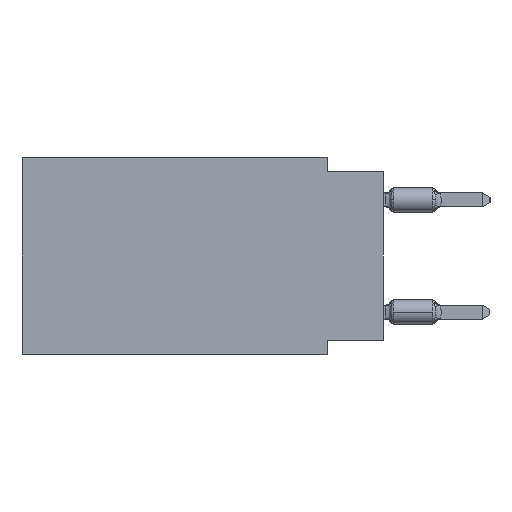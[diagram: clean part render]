
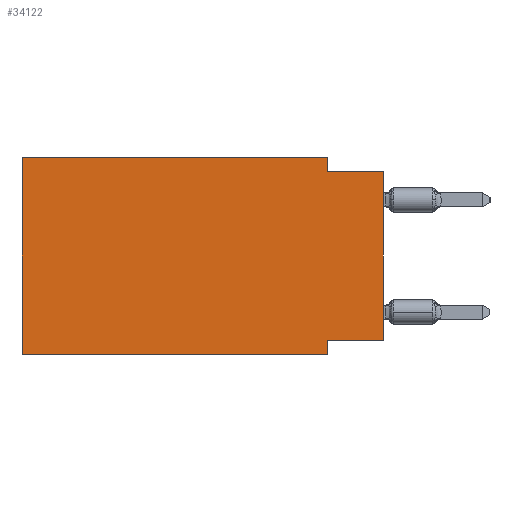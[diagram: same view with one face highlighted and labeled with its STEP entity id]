
A CAD part, left-side view. The second image highlights one B-rep face of the part: STEP entity #34122.
In plain terms, the highlighted planar face has unit normal (-1, 0, 0).
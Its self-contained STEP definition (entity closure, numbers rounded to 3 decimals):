
#1573 = DIRECTION ( 'NONE',  ( 0., 1., 0. ) ) ;
#1700 = ORIENTED_EDGE ( 'NONE', *, *, #41663, .F. ) ;
#1759 = CARTESIAN_POINT ( 'NONE',  ( 0., 0., -8.255 ) ) ;
#2011 = ORIENTED_EDGE ( 'NONE', *, *, #25797, .F. ) ;
#2292 = EDGE_CURVE ( 'NONE', #13753, #52711, #33575, .T. ) ;
#4711 = CARTESIAN_POINT ( 'NONE',  ( 0., 2.54, -8.255 ) ) ;
#5751 = EDGE_CURVE ( 'NONE', #40025, #49163, #55352, .T. ) ;
#7011 = CARTESIAN_POINT ( 'NONE',  ( 0., 2.54, -8.89 ) ) ;
#7287 = VECTOR ( 'NONE', #16326, 1000. ) ;
#8347 = VERTEX_POINT ( 'NONE', #1759 ) ;
#9127 = DIRECTION ( 'NONE',  ( 0., 0., 1. ) ) ;
#9453 = VECTOR ( 'NONE', #16396, 1000. ) ;
#9945 = CARTESIAN_POINT ( 'NONE',  ( 0., 0., -8.255 ) ) ;
#10442 = EDGE_CURVE ( 'NONE', #44852, #52711, #16675, .T. ) ;
#10452 = CARTESIAN_POINT ( 'NONE',  ( 0., 16.383, 0. ) ) ;
#10719 = DIRECTION ( 'NONE',  ( 0., 0., 1. ) ) ;
#11696 = CARTESIAN_POINT ( 'NONE',  ( 0., 0., -0.635 ) ) ;
#12952 = PLANE ( 'NONE',  #20829 ) ;
#12977 = CARTESIAN_POINT ( 'NONE',  ( 0., 0., -0.635 ) ) ;
#13419 = LINE ( 'NONE', #52734, #39937 ) ;
#13753 = VERTEX_POINT ( 'NONE', #4711 ) ;
#15290 = CARTESIAN_POINT ( 'NONE',  ( 0., 2.54, -0.635 ) ) ;
#16326 = DIRECTION ( 'NONE',  ( 0., -1., 0. ) ) ;
#16396 = DIRECTION ( 'NONE',  ( 0., -1., 0. ) ) ;
#16675 = LINE ( 'NONE', #55991, #9453 ) ;
#17977 = VECTOR ( 'NONE', #9127, 1000. ) ;
#18439 = DIRECTION ( 'NONE',  ( 0., 0., -1. ) ) ;
#18718 = DIRECTION ( 'NONE',  ( 0., 0., -1. ) ) ;
#20015 = DIRECTION ( 'NONE',  ( 0., 0., -1. ) ) ;
#20829 = AXIS2_PLACEMENT_3D ( 'NONE', #30554, #48190, #18439 ) ;
#21180 = VERTEX_POINT ( 'NONE', #10452 ) ;
#21572 = EDGE_LOOP ( 'NONE', ( #53110, #41606, #1700, #54031, #53590, #26349, #45140, #2011 ) ) ;
#25103 = FACE_OUTER_BOUND ( 'NONE', #21572, .T. ) ;
#25797 = EDGE_CURVE ( 'NONE', #8347, #13753, #36219, .T. ) ;
#26244 = VECTOR ( 'NONE', #18718, 1000. ) ;
#26349 = ORIENTED_EDGE ( 'NONE', *, *, #10442, .T. ) ;
#26803 = VECTOR ( 'NONE', #1573, 1000. ) ;
#28855 = CARTESIAN_POINT ( 'NONE',  ( 0., 16.383, -8.89 ) ) ;
#29583 = EDGE_CURVE ( 'NONE', #21180, #52968, #13419, .T. ) ;
#29989 = EDGE_CURVE ( 'NONE', #8347, #49163, #54381, .T. ) ;
#30554 = CARTESIAN_POINT ( 'NONE',  ( 0., 16.383, 0. ) ) ;
#31038 = DIRECTION ( 'NONE',  ( 0., -1., 0. ) ) ;
#31064 = CARTESIAN_POINT ( 'NONE',  ( 0., 16.383, 0. ) ) ;
#33575 = LINE ( 'NONE', #7011, #34655 ) ;
#34122 = ADVANCED_FACE ( 'NONE', ( #25103 ), #12952, .F. ) ;
#34655 = VECTOR ( 'NONE', #20015, 1000. ) ;
#34838 = LINE ( 'NONE', #31064, #17977 ) ;
#36219 = LINE ( 'NONE', #9945, #26803 ) ;
#39937 = VECTOR ( 'NONE', #31038, 1000. ) ;
#40025 = VERTEX_POINT ( 'NONE', #15290 ) ;
#40086 = CARTESIAN_POINT ( 'NONE',  ( 0., 2.54, 0. ) ) ;
#40671 = LINE ( 'NONE', #40086, #26244 ) ;
#41306 = CARTESIAN_POINT ( 'NONE',  ( 0., 2.54, -8.89 ) ) ;
#41606 = ORIENTED_EDGE ( 'NONE', *, *, #5751, .F. ) ;
#41663 = EDGE_CURVE ( 'NONE', #52968, #40025, #40671, .T. ) ;
#44852 = VERTEX_POINT ( 'NONE', #28855 ) ;
#45140 = ORIENTED_EDGE ( 'NONE', *, *, #2292, .F. ) ;
#46075 = CARTESIAN_POINT ( 'NONE',  ( 0., 2.54, 0. ) ) ;
#48160 = VECTOR ( 'NONE', #10719, 1000. ) ;
#48190 = DIRECTION ( 'NONE',  ( 1., 0., 0. ) ) ;
#49163 = VERTEX_POINT ( 'NONE', #12977 ) ;
#52711 = VERTEX_POINT ( 'NONE', #41306 ) ;
#52734 = CARTESIAN_POINT ( 'NONE',  ( 0., 16.383, 0. ) ) ;
#52968 = VERTEX_POINT ( 'NONE', #46075 ) ;
#53110 = ORIENTED_EDGE ( 'NONE', *, *, #29989, .T. ) ;
#53590 = ORIENTED_EDGE ( 'NONE', *, *, #55496, .F. ) ;
#54031 = ORIENTED_EDGE ( 'NONE', *, *, #29583, .F. ) ;
#54381 = LINE ( 'NONE', #54652, #48160 ) ;
#54652 = CARTESIAN_POINT ( 'NONE',  ( 0., 0., 0. ) ) ;
#55352 = LINE ( 'NONE', #11696, #7287 ) ;
#55496 = EDGE_CURVE ( 'NONE', #44852, #21180, #34838, .T. ) ;
#55991 = CARTESIAN_POINT ( 'NONE',  ( 0., 16.383, -8.89 ) ) ;
